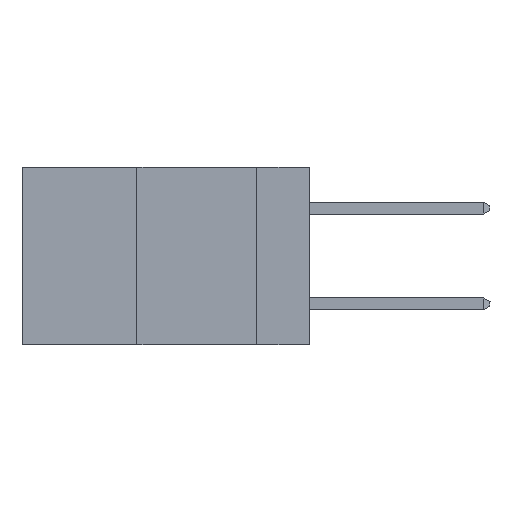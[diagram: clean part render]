
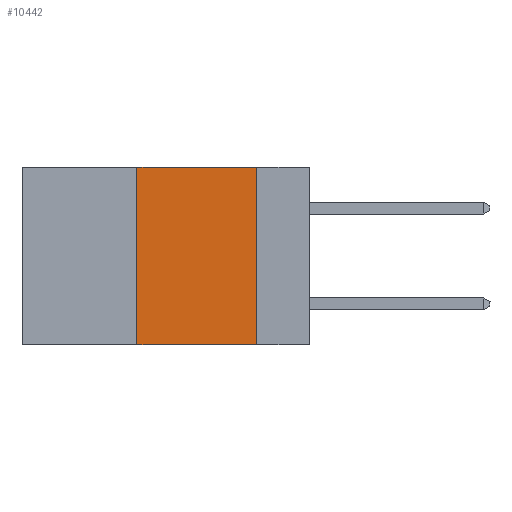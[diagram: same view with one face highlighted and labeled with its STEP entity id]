
A CAD part, left-side view. The second image highlights one B-rep face of the part: STEP entity #10442.
In plain terms, the highlighted planar face has unit normal (-1, 0, 0).
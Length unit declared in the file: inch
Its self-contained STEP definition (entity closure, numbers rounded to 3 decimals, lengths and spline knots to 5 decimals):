
#1360 = EDGE_LOOP ( 'NONE', ( #19428, #27044, #12250, #12960 ) ) ;
#1864 = CARTESIAN_POINT ( 'NONE',  ( 0., 0.36, 0. ) ) ;
#1898 = VERTEX_POINT ( 'NONE', #9371 ) ;
#2765 = VECTOR ( 'NONE', #8037, 39.37008 ) ;
#3393 = FACE_OUTER_BOUND ( 'NONE', #1360, .T. ) ;
#5421 = DIRECTION ( 'NONE',  ( 0., 0., -1. ) ) ;
#5876 = CARTESIAN_POINT ( 'NONE',  ( 0., 0.6, -0.37 ) ) ;
#6440 = CARTESIAN_POINT ( 'NONE',  ( 0., 0.6, 0. ) ) ;
#6506 = DIRECTION ( 'NONE',  ( 0., -1., 0. ) ) ;
#7387 = CARTESIAN_POINT ( 'NONE',  ( 0., 0.11, 0. ) ) ;
#8037 = DIRECTION ( 'NONE',  ( 0., -1., 0. ) ) ;
#8416 = EDGE_CURVE ( 'NONE', #14080, #1898, #24811, .T. ) ;
#8904 = CARTESIAN_POINT ( 'NONE',  ( 0., 0.36, -0.37 ) ) ;
#9371 = CARTESIAN_POINT ( 'NONE',  ( 0., 0.11, -0.37 ) ) ;
#10442 = ADVANCED_FACE ( 'NONE', ( #3393 ), #21770, .F. ) ;
#10527 = VECTOR ( 'NONE', #19363, 39.37008 ) ;
#10643 = VERTEX_POINT ( 'NONE', #8904 ) ;
#10704 = VECTOR ( 'NONE', #6506, 39.37008 ) ;
#11530 = AXIS2_PLACEMENT_3D ( 'NONE', #6440, #13157, #15189 ) ;
#12250 = ORIENTED_EDGE ( 'NONE', *, *, #23566, .F. ) ;
#12960 = ORIENTED_EDGE ( 'NONE', *, *, #16380, .T. ) ;
#13115 = VECTOR ( 'NONE', #5421, 39.37008 ) ;
#13157 = DIRECTION ( 'NONE',  ( 1., 0., 0. ) ) ;
#14080 = VERTEX_POINT ( 'NONE', #27227 ) ;
#15189 = DIRECTION ( 'NONE',  ( 0., 0., -1. ) ) ;
#16380 = EDGE_CURVE ( 'NONE', #10643, #1898, #26140, .T. ) ;
#18513 = LINE ( 'NONE', #1864, #10527 ) ;
#19363 = DIRECTION ( 'NONE',  ( 0., 0., 1. ) ) ;
#19428 = ORIENTED_EDGE ( 'NONE', *, *, #8416, .F. ) ;
#19703 = VERTEX_POINT ( 'NONE', #27055 ) ;
#19728 = EDGE_CURVE ( 'NONE', #19703, #14080, #20349, .T. ) ;
#20349 = LINE ( 'NONE', #26210, #10704 ) ;
#21770 = PLANE ( 'NONE',  #11530 ) ;
#23566 = EDGE_CURVE ( 'NONE', #10643, #19703, #18513, .T. ) ;
#24811 = LINE ( 'NONE', #7387, #13115 ) ;
#26140 = LINE ( 'NONE', #5876, #2765 ) ;
#26210 = CARTESIAN_POINT ( 'NONE',  ( 0., 0.6, 0. ) ) ;
#27044 = ORIENTED_EDGE ( 'NONE', *, *, #19728, .F. ) ;
#27055 = CARTESIAN_POINT ( 'NONE',  ( 0., 0.36, 0. ) ) ;
#27227 = CARTESIAN_POINT ( 'NONE',  ( 0., 0.11, 0. ) ) ;
